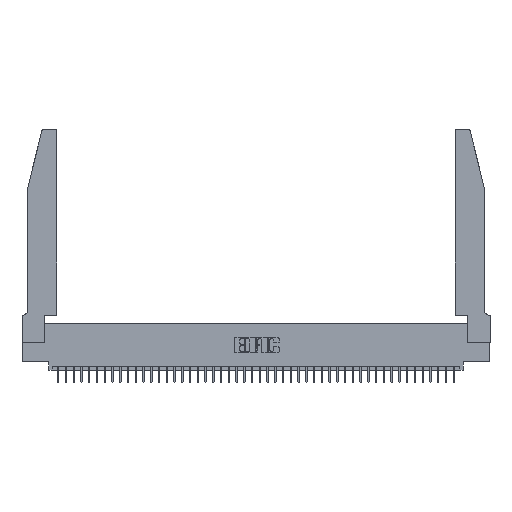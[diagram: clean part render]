
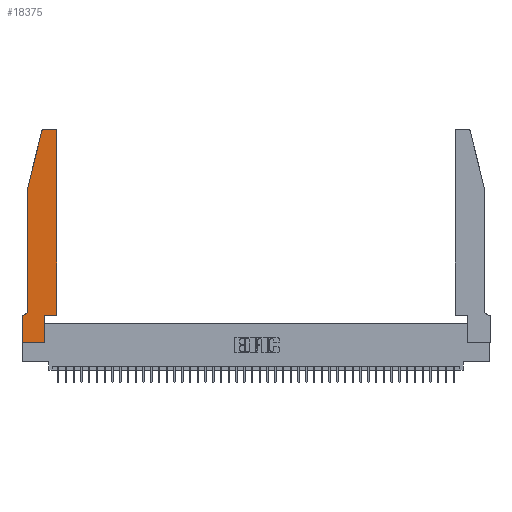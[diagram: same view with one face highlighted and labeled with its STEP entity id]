
A CAD part, top view. The second image highlights one B-rep face of the part: STEP entity #18375.
In plain terms, the highlighted planar face has unit normal (0, 0, 1).
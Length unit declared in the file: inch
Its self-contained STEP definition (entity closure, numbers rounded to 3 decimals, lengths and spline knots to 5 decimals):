
#358 = CARTESIAN_POINT ( 'NONE',  ( 0.0755, 0.42, 0.37 ) ) ;
#534 = AXIS2_PLACEMENT_3D ( 'NONE', #36039, #25317, #28748 ) ;
#737 = VERTEX_POINT ( 'NONE', #31781 ) ;
#1095 = EDGE_CURVE ( 'NONE', #737, #2203, #21341, .T. ) ;
#1755 = DIRECTION ( 'NONE',  ( 0., -1., 0. ) ) ;
#1763 = ORIENTED_EDGE ( 'NONE', *, *, #32920, .T. ) ;
#1835 = DIRECTION ( 'NONE',  ( 1., 0., 0. ) ) ;
#2203 = VERTEX_POINT ( 'NONE', #5406 ) ;
#2225 = VECTOR ( 'NONE', #18086, 39.37008 ) ;
#2423 = VECTOR ( 'NONE', #23148, 39.37008 ) ;
#2606 = VERTEX_POINT ( 'NONE', #34467 ) ;
#2731 = DIRECTION ( 'NONE',  ( 0., -1., 0. ) ) ;
#2807 = CIRCLE ( 'NONE', #14053, 0.03 ) ;
#3346 = VERTEX_POINT ( 'NONE', #21404 ) ;
#4429 = VERTEX_POINT ( 'NONE', #28209 ) ;
#4534 = LINE ( 'NONE', #4843, #2423 ) ;
#4843 = CARTESIAN_POINT ( 'NONE',  ( 0.2605, 2.75, 0.37 ) ) ;
#5389 = DIRECTION ( 'NONE',  ( 1., 0., 0. ) ) ;
#5406 = CARTESIAN_POINT ( 'NONE',  ( 0.2865, 0.35, 0.37 ) ) ;
#5634 = CARTESIAN_POINT ( 'NONE',  ( 0.0755, 0.35, 0.37 ) ) ;
#5639 = EDGE_CURVE ( 'NONE', #4429, #3346, #13948, .T. ) ;
#6295 = EDGE_CURVE ( 'NONE', #37812, #9801, #44063, .T. ) ;
#7242 = EDGE_CURVE ( 'NONE', #2606, #11790, #2807, .T. ) ;
#8477 = CARTESIAN_POINT ( 'NONE',  ( 0., 0., 0.37 ) ) ;
#8942 = EDGE_CURVE ( 'NONE', #44114, #14050, #37619, .T. ) ;
#9801 = VERTEX_POINT ( 'NONE', #33736 ) ;
#9906 = VECTOR ( 'NONE', #5389, 39.37008 ) ;
#10143 = CARTESIAN_POINT ( 'NONE',  ( 0.0055, 0.42, 0.37 ) ) ;
#10739 = VECTOR ( 'NONE', #24819, 39.37008 ) ;
#11790 = VERTEX_POINT ( 'NONE', #25059 ) ;
#12033 = EDGE_CURVE ( 'NONE', #2203, #4429, #26111, .T. ) ;
#13028 = DIRECTION ( 'NONE',  ( 0., 1., 0. ) ) ;
#13405 = FACE_OUTER_BOUND ( 'NONE', #19385, .T. ) ;
#13676 = VECTOR ( 'NONE', #16423, 39.37008 ) ;
#13948 = LINE ( 'NONE', #30926, #2225 ) ;
#14050 = VERTEX_POINT ( 'NONE', #14429 ) ;
#14053 = AXIS2_PLACEMENT_3D ( 'NONE', #33456, #19748, #24076 ) ;
#14320 = ORIENTED_EDGE ( 'NONE', *, *, #25950, .T. ) ;
#14429 = CARTESIAN_POINT ( 'NONE',  ( 0.0055, 0.35, 0.37 ) ) ;
#14733 = ORIENTED_EDGE ( 'NONE', *, *, #44360, .T. ) ;
#14951 = VECTOR ( 'NONE', #1755, 39.37008 ) ;
#15877 = VERTEX_POINT ( 'NONE', #16619 ) ;
#16423 = DIRECTION ( 'NONE',  ( 1., 0., 0. ) ) ;
#16619 = CARTESIAN_POINT ( 'NONE',  ( 0.4205, 2.75, 0.37 ) ) ;
#17008 = AXIS2_PLACEMENT_3D ( 'NONE', #10143, #20691, #20397 ) ;
#17173 = CARTESIAN_POINT ( 'NONE',  ( 0., 0., 0.37 ) ) ;
#17404 = LINE ( 'NONE', #5634, #22260 ) ;
#17556 = CIRCLE ( 'NONE', #26883, 0.03 ) ;
#17628 = ORIENTED_EDGE ( 'NONE', *, *, #6295, .T. ) ;
#17682 = VECTOR ( 'NONE', #2731, 39.37008 ) ;
#18086 = DIRECTION ( 'NONE',  ( 0., 1., 0. ) ) ;
#18375 = ADVANCED_FACE ( 'NONE', ( #13405 ), #28584, .T. ) ;
#19385 = EDGE_LOOP ( 'NONE', ( #14320, #33758, #14733, #1763, #33146, #21856, #17628, #39954, #37820, #36076, #41272, #35326 ) ) ;
#19748 = DIRECTION ( 'NONE',  ( 0., 0., 1. ) ) ;
#20397 = DIRECTION ( 'NONE',  ( -1., 0., 0. ) ) ;
#20691 = DIRECTION ( 'NONE',  ( 0., 0., -1. ) ) ;
#21341 = LINE ( 'NONE', #33665, #42904 ) ;
#21404 = CARTESIAN_POINT ( 'NONE',  ( 0.4505, 2.72, 0.37 ) ) ;
#21856 = ORIENTED_EDGE ( 'NONE', *, *, #37090, .T. ) ;
#22260 = VECTOR ( 'NONE', #36500, 39.37008 ) ;
#23148 = DIRECTION ( 'NONE',  ( -1., 0., 0. ) ) ;
#24076 = DIRECTION ( 'NONE',  ( 1., 0., 0. ) ) ;
#24819 = DIRECTION ( 'NONE',  ( -0.239, -0.971, 0. ) ) ;
#25059 = CARTESIAN_POINT ( 'NONE',  ( 0.25487, 2.72718, 0.37 ) ) ;
#25317 = DIRECTION ( 'NONE',  ( 0., 0., 1. ) ) ;
#25950 = EDGE_CURVE ( 'NONE', #15877, #2606, #4534, .T. ) ;
#26111 = LINE ( 'NONE', #28712, #13676 ) ;
#26883 = AXIS2_PLACEMENT_3D ( 'NONE', #29309, #32634, #1835 ) ;
#28209 = CARTESIAN_POINT ( 'NONE',  ( 0.4505, 0.35, 0.37 ) ) ;
#28584 = PLANE ( 'NONE',  #534 ) ;
#28712 = CARTESIAN_POINT ( 'NONE',  ( 0.4505, 0.35, 0.37 ) ) ;
#28748 = DIRECTION ( 'NONE',  ( 1., 0., 0. ) ) ;
#29309 = CARTESIAN_POINT ( 'NONE',  ( 0.4205, 2.72, 0.37 ) ) ;
#30926 = CARTESIAN_POINT ( 'NONE',  ( 0.4505, 0.35, 0.37 ) ) ;
#31781 = CARTESIAN_POINT ( 'NONE',  ( 0.2865, 0., 0.37 ) ) ;
#32634 = DIRECTION ( 'NONE',  ( 0., 0., 1. ) ) ;
#32920 = EDGE_CURVE ( 'NONE', #37440, #44114, #39167, .T. ) ;
#33146 = ORIENTED_EDGE ( 'NONE', *, *, #8942, .T. ) ;
#33456 = CARTESIAN_POINT ( 'NONE',  ( 0.284, 2.72, 0.37 ) ) ;
#33665 = CARTESIAN_POINT ( 'NONE',  ( 0.2865, 0.35, 0.37 ) ) ;
#33702 = CARTESIAN_POINT ( 'NONE',  ( 0., 0.35, 0.37 ) ) ;
#33736 = CARTESIAN_POINT ( 'NONE',  ( 0., 0., 0.37 ) ) ;
#33758 = ORIENTED_EDGE ( 'NONE', *, *, #7242, .T. ) ;
#34467 = CARTESIAN_POINT ( 'NONE',  ( 0.284, 2.75, 0.37 ) ) ;
#35326 = ORIENTED_EDGE ( 'NONE', *, *, #35586, .T. ) ;
#35586 = EDGE_CURVE ( 'NONE', #3346, #15877, #17556, .T. ) ;
#36039 = CARTESIAN_POINT ( 'NONE',  ( 0., 0.35, 0.37 ) ) ;
#36076 = ORIENTED_EDGE ( 'NONE', *, *, #12033, .T. ) ;
#36186 = CARTESIAN_POINT ( 'NONE',  ( 0.0755, 2., 0.37 ) ) ;
#36391 = EDGE_CURVE ( 'NONE', #9801, #737, #38442, .T. ) ;
#36500 = DIRECTION ( 'NONE',  ( -1., 0., 0. ) ) ;
#37090 = EDGE_CURVE ( 'NONE', #14050, #37812, #17404, .T. ) ;
#37440 = VERTEX_POINT ( 'NONE', #38666 ) ;
#37619 = CIRCLE ( 'NONE', #17008, 0.07 ) ;
#37812 = VERTEX_POINT ( 'NONE', #33702 ) ;
#37820 = ORIENTED_EDGE ( 'NONE', *, *, #1095, .T. ) ;
#38228 = LINE ( 'NONE', #38810, #10739 ) ;
#38442 = LINE ( 'NONE', #8477, #9906 ) ;
#38666 = CARTESIAN_POINT ( 'NONE',  ( 0.0755, 2., 0.37 ) ) ;
#38810 = CARTESIAN_POINT ( 'NONE',  ( 0.0755, 2., 0.37 ) ) ;
#39167 = LINE ( 'NONE', #36186, #14951 ) ;
#39954 = ORIENTED_EDGE ( 'NONE', *, *, #36391, .T. ) ;
#41272 = ORIENTED_EDGE ( 'NONE', *, *, #5639, .T. ) ;
#42904 = VECTOR ( 'NONE', #13028, 39.37008 ) ;
#44063 = LINE ( 'NONE', #17173, #17682 ) ;
#44114 = VERTEX_POINT ( 'NONE', #358 ) ;
#44360 = EDGE_CURVE ( 'NONE', #11790, #37440, #38228, .T. ) ;
